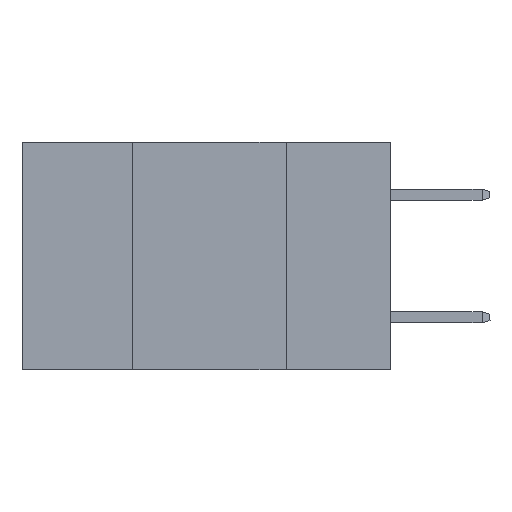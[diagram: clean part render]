
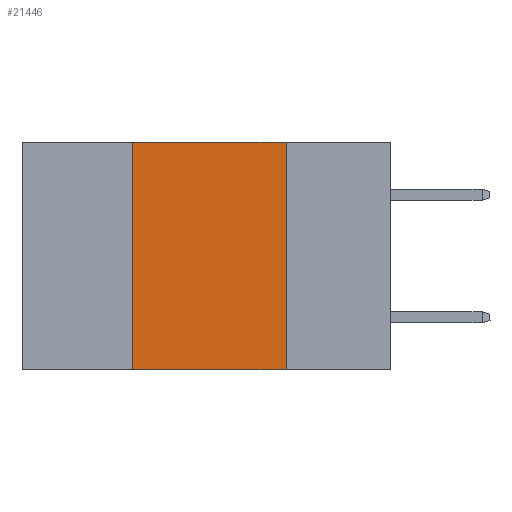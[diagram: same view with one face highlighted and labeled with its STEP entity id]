
A CAD part, left-side view. The second image highlights one B-rep face of the part: STEP entity #21446.
In plain terms, the highlighted planar face has unit normal (-1, 0, 0).
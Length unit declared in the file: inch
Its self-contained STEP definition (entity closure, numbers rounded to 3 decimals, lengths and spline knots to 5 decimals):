
#50 = AXIS2_PLACEMENT_3D ( 'NONE', #19199, #20935, #10848 ) ;
#297 = EDGE_CURVE ( 'NONE', #12845, #10901, #6888, .T. ) ;
#2750 = DIRECTION ( 'NONE',  ( 0., 0., -1. ) ) ;
#2959 = CARTESIAN_POINT ( 'NONE',  ( 0., 0.42, 0. ) ) ;
#3611 = VERTEX_POINT ( 'NONE', #2959 ) ;
#4363 = LINE ( 'NONE', #5725, #8335 ) ;
#5454 = CARTESIAN_POINT ( 'NONE',  ( 0., 0.42, 0. ) ) ;
#5725 = CARTESIAN_POINT ( 'NONE',  ( 0., 0.6, -0.37 ) ) ;
#6228 = CARTESIAN_POINT ( 'NONE',  ( 0., 0.17, 0. ) ) ;
#6284 = LINE ( 'NONE', #18592, #14673 ) ;
#6888 = LINE ( 'NONE', #16269, #19740 ) ;
#8285 = ORIENTED_EDGE ( 'NONE', *, *, #19970, .F. ) ;
#8335 = VECTOR ( 'NONE', #15769, 39.37008 ) ;
#8621 = LINE ( 'NONE', #5454, #17016 ) ;
#10848 = DIRECTION ( 'NONE',  ( 0., 0., -1. ) ) ;
#10901 = VERTEX_POINT ( 'NONE', #17794 ) ;
#10946 = ORIENTED_EDGE ( 'NONE', *, *, #16680, .T. ) ;
#11913 = DIRECTION ( 'NONE',  ( 0., -1., 0. ) ) ;
#12845 = VERTEX_POINT ( 'NONE', #6228 ) ;
#14673 = VECTOR ( 'NONE', #11913, 39.37008 ) ;
#14865 = FACE_OUTER_BOUND ( 'NONE', #15935, .T. ) ;
#15769 = DIRECTION ( 'NONE',  ( 0., -1., 0. ) ) ;
#15827 = PLANE ( 'NONE',  #50 ) ;
#15935 = EDGE_LOOP ( 'NONE', ( #20845, #8285, #20128, #10946 ) ) ;
#16269 = CARTESIAN_POINT ( 'NONE',  ( 0., 0.17, 0. ) ) ;
#16607 = CARTESIAN_POINT ( 'NONE',  ( 0., 0.42, -0.37 ) ) ;
#16680 = EDGE_CURVE ( 'NONE', #17743, #10901, #4363, .T. ) ;
#17016 = VECTOR ( 'NONE', #18877, 39.37008 ) ;
#17743 = VERTEX_POINT ( 'NONE', #16607 ) ;
#17794 = CARTESIAN_POINT ( 'NONE',  ( 0., 0.17, -0.37 ) ) ;
#18592 = CARTESIAN_POINT ( 'NONE',  ( 0., 0.6, 0. ) ) ;
#18877 = DIRECTION ( 'NONE',  ( 0., 0., 1. ) ) ;
#19199 = CARTESIAN_POINT ( 'NONE',  ( 0., 0.6, 0. ) ) ;
#19740 = VECTOR ( 'NONE', #2750, 39.37008 ) ;
#19970 = EDGE_CURVE ( 'NONE', #3611, #12845, #6284, .T. ) ;
#20077 = EDGE_CURVE ( 'NONE', #17743, #3611, #8621, .T. ) ;
#20128 = ORIENTED_EDGE ( 'NONE', *, *, #20077, .F. ) ;
#20845 = ORIENTED_EDGE ( 'NONE', *, *, #297, .F. ) ;
#20935 = DIRECTION ( 'NONE',  ( 1., 0., 0. ) ) ;
#21446 = ADVANCED_FACE ( 'NONE', ( #14865 ), #15827, .F. ) ;
